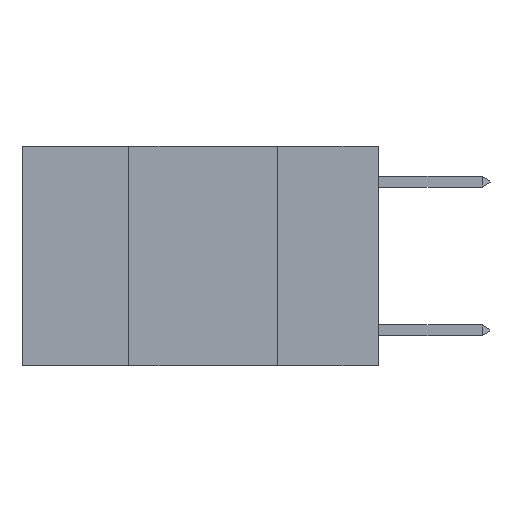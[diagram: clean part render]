
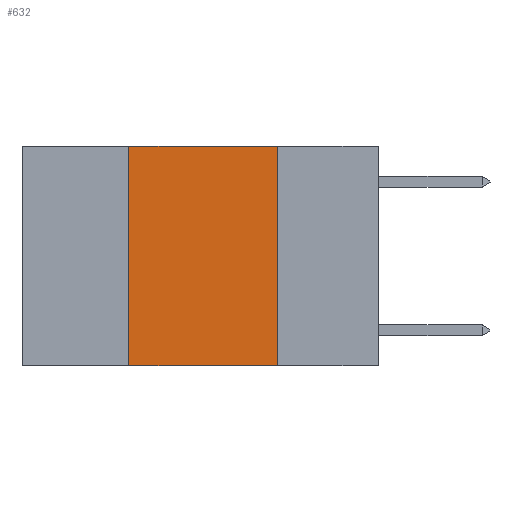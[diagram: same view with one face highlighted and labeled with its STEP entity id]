
A CAD part, left-side view. The second image highlights one B-rep face of the part: STEP entity #632.
In plain terms, the highlighted planar face has unit normal (-1, 0, 0).
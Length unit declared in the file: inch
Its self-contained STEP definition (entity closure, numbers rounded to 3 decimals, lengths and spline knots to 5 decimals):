
#468 = CARTESIAN_POINT ( 'NONE',  ( 0., 0.6, -0.37 ) ) ;
#632 = ADVANCED_FACE ( 'NONE', ( #9424 ), #702, .F. ) ;
#702 = PLANE ( 'NONE',  #10308 ) ;
#938 = EDGE_CURVE ( 'NONE', #1074, #5754, #4696, .T. ) ;
#1074 = VERTEX_POINT ( 'NONE', #8934 ) ;
#1352 = LINE ( 'NONE', #468, #9474 ) ;
#1462 = ORIENTED_EDGE ( 'NONE', *, *, #938, .F. ) ;
#1566 = VECTOR ( 'NONE', #8599, 39.37008 ) ;
#2723 = DIRECTION ( 'NONE',  ( 0., 0., 1. ) ) ;
#2998 = VERTEX_POINT ( 'NONE', #3531 ) ;
#3311 = VERTEX_POINT ( 'NONE', #11969 ) ;
#3531 = CARTESIAN_POINT ( 'NONE',  ( 0., 0.42, -0.37 ) ) ;
#3950 = EDGE_LOOP ( 'NONE', ( #1462, #12011, #11208, #7036 ) ) ;
#4679 = CARTESIAN_POINT ( 'NONE',  ( 0., 0.42, 0. ) ) ;
#4696 = LINE ( 'NONE', #8576, #9523 ) ;
#4719 = CARTESIAN_POINT ( 'NONE',  ( 0., 0.6, 0. ) ) ;
#5754 = VERTEX_POINT ( 'NONE', #12530 ) ;
#5862 = VECTOR ( 'NONE', #2723, 39.37008 ) ;
#7036 = ORIENTED_EDGE ( 'NONE', *, *, #8581, .T. ) ;
#7605 = DIRECTION ( 'NONE',  ( 0., 0., -1. ) ) ;
#8479 = CARTESIAN_POINT ( 'NONE',  ( 0., 0.6, 0. ) ) ;
#8576 = CARTESIAN_POINT ( 'NONE',  ( 0., 0.17, 0. ) ) ;
#8581 = EDGE_CURVE ( 'NONE', #2998, #5754, #1352, .T. ) ;
#8599 = DIRECTION ( 'NONE',  ( 0., -1., 0. ) ) ;
#8934 = CARTESIAN_POINT ( 'NONE',  ( 0., 0.17, 0. ) ) ;
#9424 = FACE_OUTER_BOUND ( 'NONE', #3950, .T. ) ;
#9474 = VECTOR ( 'NONE', #11018, 39.37008 ) ;
#9476 = LINE ( 'NONE', #4679, #5862 ) ;
#9523 = VECTOR ( 'NONE', #7605, 39.37008 ) ;
#9697 = EDGE_CURVE ( 'NONE', #3311, #1074, #9713, .T. ) ;
#9713 = LINE ( 'NONE', #4719, #1566 ) ;
#10308 = AXIS2_PLACEMENT_3D ( 'NONE', #8479, #11375, #10900 ) ;
#10504 = EDGE_CURVE ( 'NONE', #2998, #3311, #9476, .T. ) ;
#10900 = DIRECTION ( 'NONE',  ( 0., 0., -1. ) ) ;
#11018 = DIRECTION ( 'NONE',  ( 0., -1., 0. ) ) ;
#11208 = ORIENTED_EDGE ( 'NONE', *, *, #10504, .F. ) ;
#11375 = DIRECTION ( 'NONE',  ( 1., 0., 0. ) ) ;
#11969 = CARTESIAN_POINT ( 'NONE',  ( 0., 0.42, 0. ) ) ;
#12011 = ORIENTED_EDGE ( 'NONE', *, *, #9697, .F. ) ;
#12530 = CARTESIAN_POINT ( 'NONE',  ( 0., 0.17, -0.37 ) ) ;
